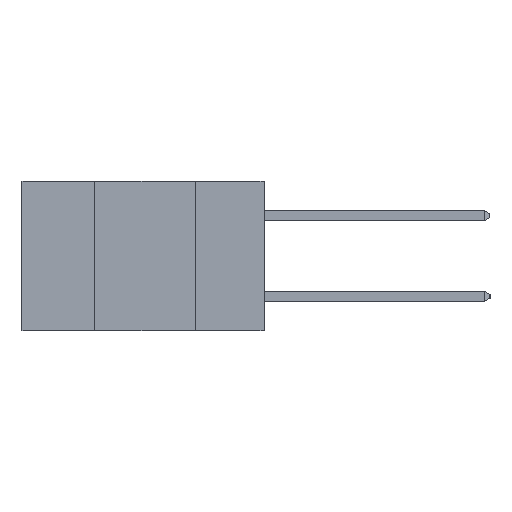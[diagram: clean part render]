
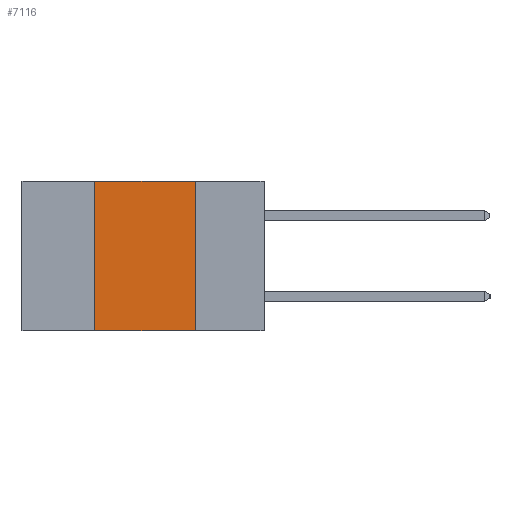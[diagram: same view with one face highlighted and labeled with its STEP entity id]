
A CAD part, left-side view. The second image highlights one B-rep face of the part: STEP entity #7116.
In plain terms, the highlighted planar face has unit normal (-1, 0, 0).
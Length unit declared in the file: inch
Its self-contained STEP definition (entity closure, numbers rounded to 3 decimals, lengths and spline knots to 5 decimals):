
#233 = FACE_OUTER_BOUND ( 'NONE', #5459, .T. ) ;
#669 = CARTESIAN_POINT ( 'NONE',  ( 0., 0.42, -0.37 ) ) ;
#1401 = VECTOR ( 'NONE', #12008, 39.37008 ) ;
#1641 = VERTEX_POINT ( 'NONE', #3490 ) ;
#1818 = CARTESIAN_POINT ( 'NONE',  ( 0., 0.17, -0.37 ) ) ;
#2189 = EDGE_CURVE ( 'NONE', #1641, #10746, #10600, .T. ) ;
#2261 = PLANE ( 'NONE',  #3444 ) ;
#3444 = AXIS2_PLACEMENT_3D ( 'NONE', #3514, #12311, #4791 ) ;
#3490 = CARTESIAN_POINT ( 'NONE',  ( 0., 0.17, 0. ) ) ;
#3514 = CARTESIAN_POINT ( 'NONE',  ( 0., 0.6, 0. ) ) ;
#4747 = LINE ( 'NONE', #669, #1401 ) ;
#4791 = DIRECTION ( 'NONE',  ( 0., 0., -1. ) ) ;
#5426 = ORIENTED_EDGE ( 'NONE', *, *, #13912, .F. ) ;
#5459 = EDGE_LOOP ( 'NONE', ( #13492, #5426, #10348, #8356 ) ) ;
#6140 = CARTESIAN_POINT ( 'NONE',  ( 0., 0.6, 0. ) ) ;
#6746 = VECTOR ( 'NONE', #11206, 39.37008 ) ;
#6824 = VECTOR ( 'NONE', #12480, 39.37008 ) ;
#7116 = ADVANCED_FACE ( 'NONE', ( #233 ), #2261, .F. ) ;
#8356 = ORIENTED_EDGE ( 'NONE', *, *, #16058, .T. ) ;
#8409 = EDGE_CURVE ( 'NONE', #8953, #8799, #4747, .T. ) ;
#8689 = CARTESIAN_POINT ( 'NONE',  ( 0., 0.17, -0.37 ) ) ;
#8799 = VERTEX_POINT ( 'NONE', #10462 ) ;
#8953 = VERTEX_POINT ( 'NONE', #13483 ) ;
#9947 = CARTESIAN_POINT ( 'NONE',  ( 0., 0.6, -0.37 ) ) ;
#10202 = VECTOR ( 'NONE', #13455, 39.37008 ) ;
#10348 = ORIENTED_EDGE ( 'NONE', *, *, #8409, .F. ) ;
#10462 = CARTESIAN_POINT ( 'NONE',  ( 0., 0.42, 0. ) ) ;
#10600 = LINE ( 'NONE', #8689, #10202 ) ;
#10746 = VERTEX_POINT ( 'NONE', #1818 ) ;
#11206 = DIRECTION ( 'NONE',  ( 0., -1., 0. ) ) ;
#12008 = DIRECTION ( 'NONE',  ( 0., 0., 1. ) ) ;
#12311 = DIRECTION ( 'NONE',  ( 1., 0., 0. ) ) ;
#12480 = DIRECTION ( 'NONE',  ( 0., -1., 0. ) ) ;
#13155 = LINE ( 'NONE', #6140, #6824 ) ;
#13455 = DIRECTION ( 'NONE',  ( 0., 0., -1. ) ) ;
#13473 = LINE ( 'NONE', #9947, #6746 ) ;
#13483 = CARTESIAN_POINT ( 'NONE',  ( 0., 0.42, -0.37 ) ) ;
#13492 = ORIENTED_EDGE ( 'NONE', *, *, #2189, .F. ) ;
#13912 = EDGE_CURVE ( 'NONE', #8799, #1641, #13155, .T. ) ;
#16058 = EDGE_CURVE ( 'NONE', #8953, #10746, #13473, .T. ) ;
